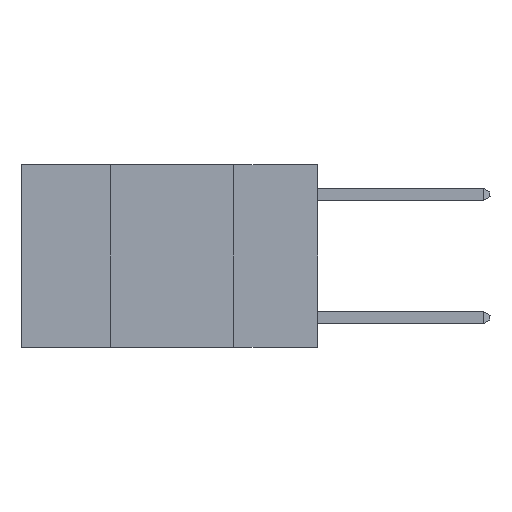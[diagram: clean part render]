
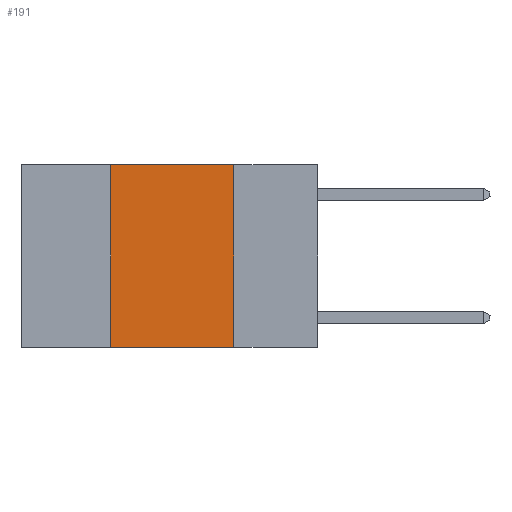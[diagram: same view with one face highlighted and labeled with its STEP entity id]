
A CAD part, left-side view. The second image highlights one B-rep face of the part: STEP entity #191.
In plain terms, the highlighted planar face has unit normal (-1, 0, 0).
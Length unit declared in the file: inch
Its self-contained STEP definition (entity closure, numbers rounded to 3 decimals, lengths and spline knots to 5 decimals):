
#191 = ADVANCED_FACE ( 'NONE', ( #5474 ), #7657, .F. ) ;
#695 = DIRECTION ( 'NONE',  ( 0., 0., -1. ) ) ;
#697 = ORIENTED_EDGE ( 'NONE', *, *, #2660, .F. ) ;
#1336 = VECTOR ( 'NONE', #11592, 39.37008 ) ;
#1473 = VECTOR ( 'NONE', #695, 39.37008 ) ;
#1499 = LINE ( 'NONE', #3391, #1336 ) ;
#1511 = ORIENTED_EDGE ( 'NONE', *, *, #6683, .F. ) ;
#2289 = LINE ( 'NONE', #3563, #2777 ) ;
#2660 = EDGE_CURVE ( 'NONE', #10080, #3208, #10142, .T. ) ;
#2777 = VECTOR ( 'NONE', #11507, 39.37008 ) ;
#3016 = EDGE_CURVE ( 'NONE', #3208, #9863, #3848, .T. ) ;
#3208 = VERTEX_POINT ( 'NONE', #5062 ) ;
#3387 = CARTESIAN_POINT ( 'NONE',  ( 0., 0.6, 0. ) ) ;
#3391 = CARTESIAN_POINT ( 'NONE',  ( 0., 0.42, 0. ) ) ;
#3517 = DIRECTION ( 'NONE',  ( 1., 0., 0. ) ) ;
#3563 = CARTESIAN_POINT ( 'NONE',  ( 0., 0.6, -0.37 ) ) ;
#3597 = VERTEX_POINT ( 'NONE', #9114 ) ;
#3695 = ORIENTED_EDGE ( 'NONE', *, *, #3016, .F. ) ;
#3848 = LINE ( 'NONE', #11982, #1473 ) ;
#4913 = EDGE_LOOP ( 'NONE', ( #3695, #697, #1511, #9075 ) ) ;
#5062 = CARTESIAN_POINT ( 'NONE',  ( 0., 0.17, 0. ) ) ;
#5474 = FACE_OUTER_BOUND ( 'NONE', #4913, .T. ) ;
#5887 = DIRECTION ( 'NONE',  ( 0., -1., 0. ) ) ;
#6683 = EDGE_CURVE ( 'NONE', #3597, #10080, #1499, .T. ) ;
#7475 = DIRECTION ( 'NONE',  ( 0., 0., -1. ) ) ;
#7657 = PLANE ( 'NONE',  #8258 ) ;
#7873 = CARTESIAN_POINT ( 'NONE',  ( 0., 0.6, 0. ) ) ;
#8258 = AXIS2_PLACEMENT_3D ( 'NONE', #3387, #3517, #7475 ) ;
#9075 = ORIENTED_EDGE ( 'NONE', *, *, #12075, .T. ) ;
#9114 = CARTESIAN_POINT ( 'NONE',  ( 0., 0.42, -0.37 ) ) ;
#9597 = VECTOR ( 'NONE', #5887, 39.37008 ) ;
#9863 = VERTEX_POINT ( 'NONE', #11472 ) ;
#10080 = VERTEX_POINT ( 'NONE', #12054 ) ;
#10142 = LINE ( 'NONE', #7873, #9597 ) ;
#11472 = CARTESIAN_POINT ( 'NONE',  ( 0., 0.17, -0.37 ) ) ;
#11507 = DIRECTION ( 'NONE',  ( 0., -1., 0. ) ) ;
#11592 = DIRECTION ( 'NONE',  ( 0., 0., 1. ) ) ;
#11982 = CARTESIAN_POINT ( 'NONE',  ( 0., 0.17, 0. ) ) ;
#12054 = CARTESIAN_POINT ( 'NONE',  ( 0., 0.42, 0. ) ) ;
#12075 = EDGE_CURVE ( 'NONE', #3597, #9863, #2289, .T. ) ;
